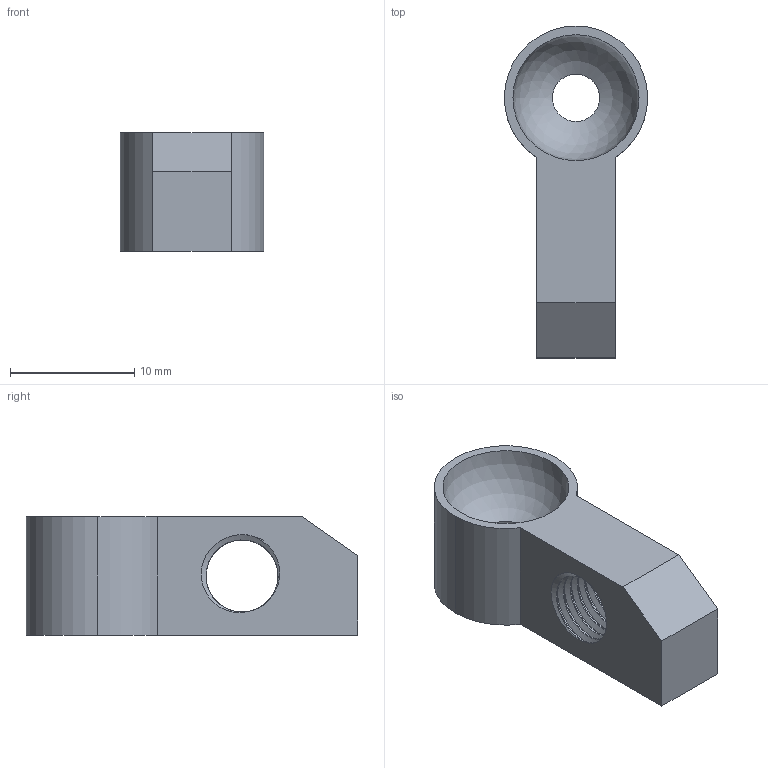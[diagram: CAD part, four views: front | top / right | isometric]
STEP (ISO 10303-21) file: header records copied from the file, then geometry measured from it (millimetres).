
FILE_DESCRIPTION (( 'STEP AP203' ), '1' );
FILE_NAME ('AF-WF-GS-PRT-008-STEP.STEP', '2020-07-21T22:58:13', ( '' ), ( '' ), 'SwSTEP 2.0', 'SolidWorks 2018', '' );
FILE_SCHEMA (( 'CONFIG_CONTROL_DESIGN' ));
Length unit declared in the file: inch
Products named in the file (1): AF-WF-GS-PRT-008-STEP
Bounding box: 11.55 x 26.73 x 9.53 mm (x, y, z)
Volume: 1362.1 mm3; surface area: 1280.2 mm2
Topology: 1 solids, 1 shells, 35 faces, 97 edges, 64 vertices
Faces by surface type: cylinder 23, plane 6, bspline 3, cone 2, sphere 1
Entity records: 4224 total; most frequent: CARTESIAN_POINT 3340, ORIENTED_EDGE 192, DIRECTION 138, EDGE_CURVE 96, VERTEX_POINT 64, AXIS2_PLACEMENT_3D 51, EDGE_LOOP 40, LINE 36
